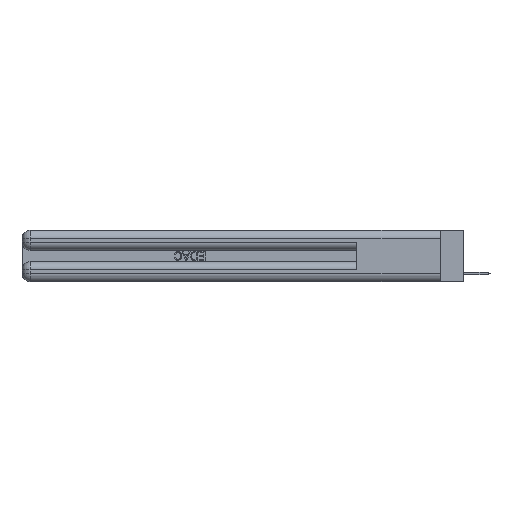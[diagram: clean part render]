
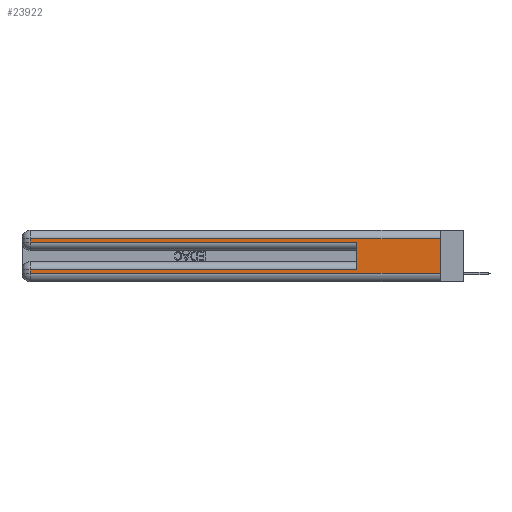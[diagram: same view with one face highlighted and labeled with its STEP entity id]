
A CAD part, left-side view. The second image highlights one B-rep face of the part: STEP entity #23922.
In plain terms, the highlighted planar face has unit normal (-1, 0, 0).
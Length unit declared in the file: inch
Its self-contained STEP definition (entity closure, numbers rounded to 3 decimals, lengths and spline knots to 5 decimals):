
#523 = DIRECTION ( 'NONE',  ( 0., 0., -1. ) ) ;
#1140 = VECTOR ( 'NONE', #23284, 39.37008 ) ;
#1564 = ORIENTED_EDGE ( 'NONE', *, *, #23815, .T. ) ;
#1579 = CARTESIAN_POINT ( 'NONE',  ( 0., 0., 0.085 ) ) ;
#2625 = DIRECTION ( 'NONE',  ( 1., 0., 0. ) ) ;
#4838 = CARTESIAN_POINT ( 'NONE',  ( 0., 2.94, 0.37 ) ) ;
#4939 = EDGE_CURVE ( 'NONE', #28607, #11784, #14672, .T. ) ;
#5055 = CARTESIAN_POINT ( 'NONE',  ( 0., 2.94, 0.37 ) ) ;
#5259 = FACE_OUTER_BOUND ( 'NONE', #21051, .T. ) ;
#5427 = CARTESIAN_POINT ( 'NONE',  ( 0., 0., 0.31 ) ) ;
#6013 = ORIENTED_EDGE ( 'NONE', *, *, #21068, .T. ) ;
#7662 = LINE ( 'NONE', #10278, #1140 ) ;
#8318 = VECTOR ( 'NONE', #19613, 39.37008 ) ;
#8790 = AXIS2_PLACEMENT_3D ( 'NONE', #21453, #2625, #9451 ) ;
#9451 = DIRECTION ( 'NONE',  ( 0., 0., -1. ) ) ;
#10186 = CARTESIAN_POINT ( 'NONE',  ( 0., 0., 0.06 ) ) ;
#10278 = CARTESIAN_POINT ( 'NONE',  ( 0., 0., 0.37 ) ) ;
#10958 = VERTEX_POINT ( 'NONE', #15478 ) ;
#11146 = ORIENTED_EDGE ( 'NONE', *, *, #16260, .F. ) ;
#11616 = LINE ( 'NONE', #1579, #19136 ) ;
#11784 = VERTEX_POINT ( 'NONE', #23384 ) ;
#12037 = CARTESIAN_POINT ( 'NONE',  ( 0., 0., 0.31 ) ) ;
#12626 = VECTOR ( 'NONE', #13328, 39.37008 ) ;
#12968 = VERTEX_POINT ( 'NONE', #22463 ) ;
#13328 = DIRECTION ( 'NONE',  ( 0., 0., 1. ) ) ;
#13434 = CARTESIAN_POINT ( 'NONE',  ( 0., 0.6, 0.285 ) ) ;
#13474 = LINE ( 'NONE', #23007, #12626 ) ;
#14672 = LINE ( 'NONE', #10186, #15391 ) ;
#15357 = VERTEX_POINT ( 'NONE', #13434 ) ;
#15391 = VECTOR ( 'NONE', #19287, 39.37008 ) ;
#15478 = CARTESIAN_POINT ( 'NONE',  ( 0., 2.94, 0.31 ) ) ;
#15950 = DIRECTION ( 'NONE',  ( 0., 1., 0. ) ) ;
#16260 = EDGE_CURVE ( 'NONE', #27724, #15357, #13474, .T. ) ;
#16491 = VERTEX_POINT ( 'NONE', #25921 ) ;
#17976 = EDGE_CURVE ( 'NONE', #19297, #11784, #7662, .T. ) ;
#18243 = VECTOR ( 'NONE', #19286, 39.37008 ) ;
#18518 = EDGE_CURVE ( 'NONE', #12968, #28607, #25964, .T. ) ;
#19136 = VECTOR ( 'NONE', #15950, 39.37008 ) ;
#19274 = ORIENTED_EDGE ( 'NONE', *, *, #17976, .F. ) ;
#19286 = DIRECTION ( 'NONE',  ( 0., -1., 0. ) ) ;
#19287 = DIRECTION ( 'NONE',  ( 0., -1., 0. ) ) ;
#19297 = VERTEX_POINT ( 'NONE', #12037 ) ;
#19613 = DIRECTION ( 'NONE',  ( 0., 1., 0. ) ) ;
#20440 = ORIENTED_EDGE ( 'NONE', *, *, #18518, .T. ) ;
#20636 = CARTESIAN_POINT ( 'NONE',  ( 0., 0.6, 0.085 ) ) ;
#20868 = VECTOR ( 'NONE', #523, 39.37008 ) ;
#21051 = EDGE_LOOP ( 'NONE', ( #19274, #22378, #6013, #29696, #11146, #1564, #20440, #24247 ) ) ;
#21068 = EDGE_CURVE ( 'NONE', #10958, #16491, #23395, .T. ) ;
#21453 = CARTESIAN_POINT ( 'NONE',  ( 0., 0., 0.37 ) ) ;
#21780 = LINE ( 'NONE', #5427, #8318 ) ;
#22378 = ORIENTED_EDGE ( 'NONE', *, *, #25857, .T. ) ;
#22463 = CARTESIAN_POINT ( 'NONE',  ( 0., 2.94, 0.085 ) ) ;
#23007 = CARTESIAN_POINT ( 'NONE',  ( 0., 0.6, 0.145 ) ) ;
#23284 = DIRECTION ( 'NONE',  ( 0., 0., -1. ) ) ;
#23384 = CARTESIAN_POINT ( 'NONE',  ( 0., 0., 0.06 ) ) ;
#23395 = LINE ( 'NONE', #5055, #27880 ) ;
#23444 = CARTESIAN_POINT ( 'NONE',  ( 0., 0., 0.285 ) ) ;
#23787 = PLANE ( 'NONE',  #8790 ) ;
#23815 = EDGE_CURVE ( 'NONE', #27724, #12968, #11616, .T. ) ;
#23922 = ADVANCED_FACE ( 'NONE', ( #5259 ), #23787, .F. ) ;
#24247 = ORIENTED_EDGE ( 'NONE', *, *, #4939, .T. ) ;
#25857 = EDGE_CURVE ( 'NONE', #19297, #10958, #21780, .T. ) ;
#25921 = CARTESIAN_POINT ( 'NONE',  ( 0., 2.94, 0.285 ) ) ;
#25964 = LINE ( 'NONE', #4838, #20868 ) ;
#27327 = EDGE_CURVE ( 'NONE', #16491, #15357, #28368, .T. ) ;
#27724 = VERTEX_POINT ( 'NONE', #20636 ) ;
#27880 = VECTOR ( 'NONE', #28633, 39.37008 ) ;
#27918 = CARTESIAN_POINT ( 'NONE',  ( 0., 2.94, 0.06 ) ) ;
#28368 = LINE ( 'NONE', #23444, #18243 ) ;
#28607 = VERTEX_POINT ( 'NONE', #27918 ) ;
#28633 = DIRECTION ( 'NONE',  ( 0., 0., -1. ) ) ;
#29696 = ORIENTED_EDGE ( 'NONE', *, *, #27327, .T. ) ;
